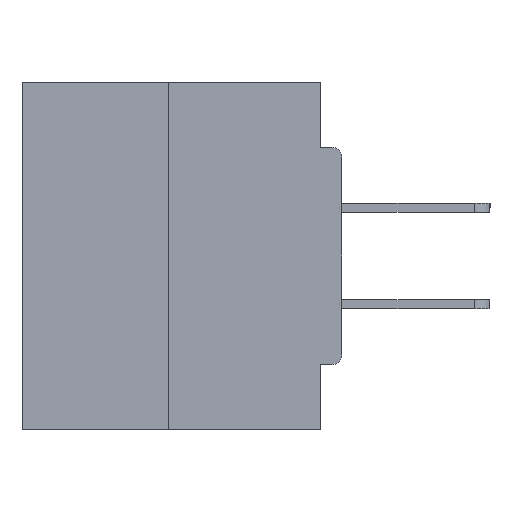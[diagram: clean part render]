
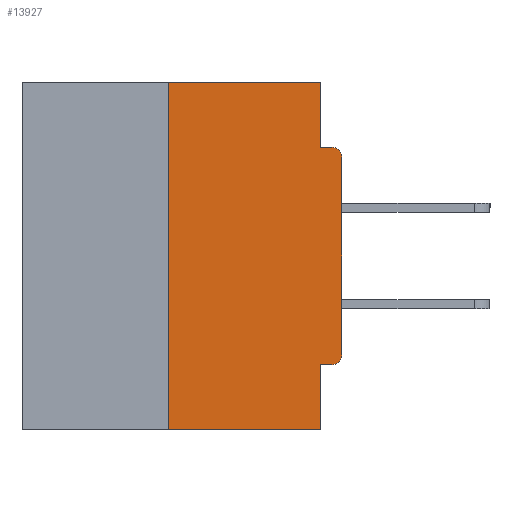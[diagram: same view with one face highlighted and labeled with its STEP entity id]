
A CAD part, left-side view. The second image highlights one B-rep face of the part: STEP entity #13927.
In plain terms, the highlighted planar face has unit normal (-1, 0, 0).
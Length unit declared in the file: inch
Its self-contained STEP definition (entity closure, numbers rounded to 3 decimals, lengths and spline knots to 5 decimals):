
#640 = EDGE_CURVE ( 'NONE', #7956, #3778, #10374, .T. ) ;
#691 = LINE ( 'NONE', #5069, #30374 ) ;
#901 = CARTESIAN_POINT ( 'NONE',  ( 0., 0.25, -0.5 ) ) ;
#903 = VECTOR ( 'NONE', #8299, 39.37008 ) ;
#1099 = CIRCLE ( 'NONE', #15459, 0.015 ) ;
#2406 = VERTEX_POINT ( 'NONE', #35286 ) ;
#2765 = EDGE_CURVE ( 'NONE', #7956, #10309, #22499, .T. ) ;
#2939 = VERTEX_POINT ( 'NONE', #5260 ) ;
#3170 = DIRECTION ( 'NONE',  ( 1., 0., 0. ) ) ;
#3778 = VERTEX_POINT ( 'NONE', #19802 ) ;
#4326 = ORIENTED_EDGE ( 'NONE', *, *, #14415, .T. ) ;
#4676 = CARTESIAN_POINT ( 'NONE',  ( 0., 0.015, -0.4065 ) ) ;
#5069 = CARTESIAN_POINT ( 'NONE',  ( 0., 0.031, -0.5 ) ) ;
#5255 = DIRECTION ( 'NONE',  ( 0., 0., 1. ) ) ;
#5260 = CARTESIAN_POINT ( 'NONE',  ( 0., 0., -0.1085 ) ) ;
#5483 = EDGE_CURVE ( 'NONE', #2406, #2939, #32505, .T. ) ;
#5823 = VECTOR ( 'NONE', #15101, 39.37008 ) ;
#6543 = DIRECTION ( 'NONE',  ( 0., 0., -1. ) ) ;
#6594 = CARTESIAN_POINT ( 'NONE',  ( 0., 0.25, 0. ) ) ;
#6834 = CARTESIAN_POINT ( 'NONE',  ( 0., 0.46, -0.5 ) ) ;
#6976 = CARTESIAN_POINT ( 'NONE',  ( 0., 0.031, -0.0935 ) ) ;
#7097 = ORIENTED_EDGE ( 'NONE', *, *, #8906, .F. ) ;
#7917 = DIRECTION ( 'NONE',  ( 0., 0., -1. ) ) ;
#7948 = VECTOR ( 'NONE', #30121, 39.37008 ) ;
#7956 = VERTEX_POINT ( 'NONE', #901 ) ;
#8299 = DIRECTION ( 'NONE',  ( 0., 1., 0. ) ) ;
#8597 = VERTEX_POINT ( 'NONE', #26004 ) ;
#8906 = EDGE_CURVE ( 'NONE', #23970, #3778, #691, .T. ) ;
#9039 = CARTESIAN_POINT ( 'NONE',  ( 0., 0., -0.0935 ) ) ;
#9177 = ORIENTED_EDGE ( 'NONE', *, *, #19298, .F. ) ;
#9221 = DIRECTION ( 'NONE',  ( 0., 0., -1. ) ) ;
#9630 = CARTESIAN_POINT ( 'NONE',  ( 0., 0.46, 0. ) ) ;
#10303 = CARTESIAN_POINT ( 'NONE',  ( 0., 0.031, 0. ) ) ;
#10309 = VERTEX_POINT ( 'NONE', #6594 ) ;
#10374 = LINE ( 'NONE', #6834, #5823 ) ;
#11256 = VECTOR ( 'NONE', #23890, 39.37008 ) ;
#11566 = CARTESIAN_POINT ( 'NONE',  ( 0., 0.46, 0. ) ) ;
#11642 = CIRCLE ( 'NONE', #18409, 0.015 ) ;
#13153 = DIRECTION ( 'NONE',  ( 0., -1., 0. ) ) ;
#13927 = ADVANCED_FACE ( 'NONE', ( #36640 ), #28789, .F. ) ;
#14112 = ORIENTED_EDGE ( 'NONE', *, *, #5483, .T. ) ;
#14415 = EDGE_CURVE ( 'NONE', #2939, #23885, #1099, .T. ) ;
#15101 = DIRECTION ( 'NONE',  ( 0., -1., 0. ) ) ;
#15445 = LINE ( 'NONE', #10303, #7948 ) ;
#15459 = AXIS2_PLACEMENT_3D ( 'NONE', #23742, #15527, #6543 ) ;
#15487 = LINE ( 'NONE', #25257, #903 ) ;
#15527 = DIRECTION ( 'NONE',  ( -1., 0., 0. ) ) ;
#16250 = ORIENTED_EDGE ( 'NONE', *, *, #30905, .F. ) ;
#16448 = EDGE_CURVE ( 'NONE', #29774, #23970, #15487, .T. ) ;
#17139 = LINE ( 'NONE', #9039, #34919 ) ;
#18409 = AXIS2_PLACEMENT_3D ( 'NONE', #27591, #19031, #7917 ) ;
#19031 = DIRECTION ( 'NONE',  ( -1., 0., 0. ) ) ;
#19272 = ORIENTED_EDGE ( 'NONE', *, *, #34466, .F. ) ;
#19298 = EDGE_CURVE ( 'NONE', #30863, #23885, #17139, .T. ) ;
#19802 = CARTESIAN_POINT ( 'NONE',  ( 0., 0.031, -0.5 ) ) ;
#20003 = DIRECTION ( 'NONE',  ( 0., 0., 1. ) ) ;
#20101 = LINE ( 'NONE', #9630, #11256 ) ;
#22499 = LINE ( 'NONE', #28920, #28699 ) ;
#23742 = CARTESIAN_POINT ( 'NONE',  ( 0., 0.015, -0.1085 ) ) ;
#23789 = ORIENTED_EDGE ( 'NONE', *, *, #28649, .T. ) ;
#23885 = VERTEX_POINT ( 'NONE', #35149 ) ;
#23890 = DIRECTION ( 'NONE',  ( 0., -1., 0. ) ) ;
#23970 = VERTEX_POINT ( 'NONE', #29298 ) ;
#24084 = VECTOR ( 'NONE', #5255, 39.37008 ) ;
#24977 = ORIENTED_EDGE ( 'NONE', *, *, #640, .T. ) ;
#25257 = CARTESIAN_POINT ( 'NONE',  ( 0., 0., -0.4065 ) ) ;
#25653 = ORIENTED_EDGE ( 'NONE', *, *, #16448, .F. ) ;
#26004 = CARTESIAN_POINT ( 'NONE',  ( 0., 0.031, 0. ) ) ;
#26850 = AXIS2_PLACEMENT_3D ( 'NONE', #11566, #3170, #9221 ) ;
#27591 = CARTESIAN_POINT ( 'NONE',  ( 0., 0.015, -0.3915 ) ) ;
#28649 = EDGE_CURVE ( 'NONE', #29774, #2406, #11642, .T. ) ;
#28699 = VECTOR ( 'NONE', #20003, 39.37008 ) ;
#28789 = PLANE ( 'NONE',  #26850 ) ;
#28920 = CARTESIAN_POINT ( 'NONE',  ( 0., 0.25, 0. ) ) ;
#29298 = CARTESIAN_POINT ( 'NONE',  ( 0., 0.031, -0.4065 ) ) ;
#29774 = VERTEX_POINT ( 'NONE', #4676 ) ;
#30121 = DIRECTION ( 'NONE',  ( 0., 0., -1. ) ) ;
#30374 = VECTOR ( 'NONE', #35656, 39.37008 ) ;
#30863 = VERTEX_POINT ( 'NONE', #6976 ) ;
#30905 = EDGE_CURVE ( 'NONE', #8597, #30863, #15445, .T. ) ;
#32505 = LINE ( 'NONE', #36464, #24084 ) ;
#33958 = ORIENTED_EDGE ( 'NONE', *, *, #2765, .F. ) ;
#34466 = EDGE_CURVE ( 'NONE', #10309, #8597, #20101, .T. ) ;
#34919 = VECTOR ( 'NONE', #13153, 39.37008 ) ;
#35149 = CARTESIAN_POINT ( 'NONE',  ( 0., 0.015, -0.0935 ) ) ;
#35286 = CARTESIAN_POINT ( 'NONE',  ( 0., 0., -0.3915 ) ) ;
#35656 = DIRECTION ( 'NONE',  ( 0., 0., -1. ) ) ;
#35702 = EDGE_LOOP ( 'NONE', ( #19272, #33958, #24977, #7097, #25653, #23789, #14112, #4326, #9177, #16250 ) ) ;
#36464 = CARTESIAN_POINT ( 'NONE',  ( 0., 0., 0. ) ) ;
#36640 = FACE_OUTER_BOUND ( 'NONE', #35702, .T. ) ;
